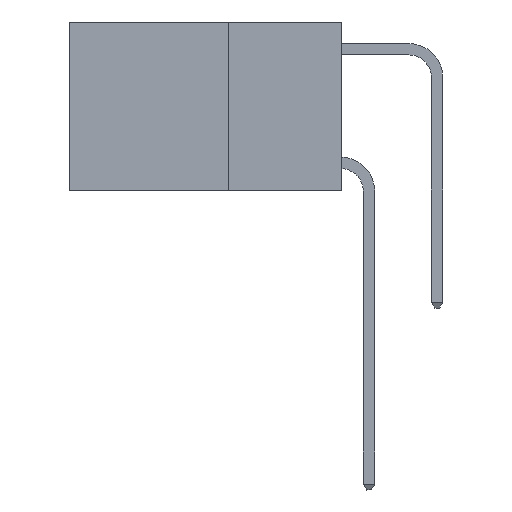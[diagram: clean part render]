
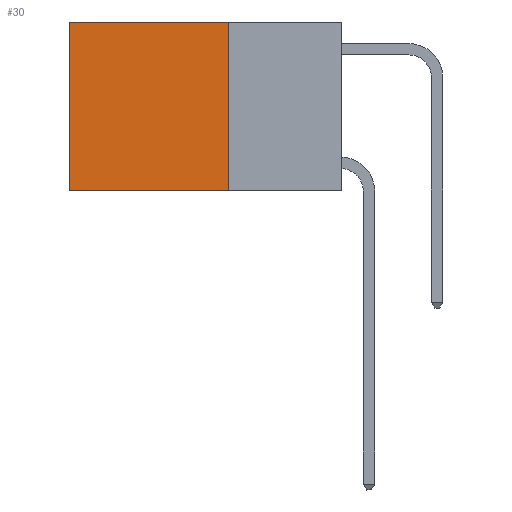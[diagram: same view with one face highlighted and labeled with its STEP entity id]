
A CAD part, left-side view. The second image highlights one B-rep face of the part: STEP entity #30.
In plain terms, the highlighted planar face has unit normal (-1, 0, 0).
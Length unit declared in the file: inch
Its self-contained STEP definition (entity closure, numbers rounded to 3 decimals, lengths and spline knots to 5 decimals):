
#30 = ADVANCED_FACE ( 'NONE', ( #6235 ), #3145, .F. ) ;
#73 = CARTESIAN_POINT ( 'NONE',  ( 0.2625, 0.25, 0. ) ) ;
#166 = DIRECTION ( 'NONE',  ( 1., 0., 0. ) ) ;
#639 = ORIENTED_EDGE ( 'NONE', *, *, #18662, .F. ) ;
#1713 = AXIS2_PLACEMENT_3D ( 'NONE', #73, #166, #11077 ) ;
#2638 = EDGE_CURVE ( 'NONE', #12230, #5429, #14148, .T. ) ;
#2720 = VERTEX_POINT ( 'NONE', #3259 ) ;
#3145 = PLANE ( 'NONE',  #1713 ) ;
#3259 = CARTESIAN_POINT ( 'NONE',  ( 0.2625, 0.6, -0.37 ) ) ;
#3732 = ORIENTED_EDGE ( 'NONE', *, *, #18533, .T. ) ;
#4660 = LINE ( 'NONE', #8150, #9643 ) ;
#4895 = ORIENTED_EDGE ( 'NONE', *, *, #7641, .F. ) ;
#5124 = LINE ( 'NONE', #6735, #8877 ) ;
#5429 = VERTEX_POINT ( 'NONE', #7804 ) ;
#6158 = DIRECTION ( 'NONE',  ( 0., 0., -1. ) ) ;
#6235 = FACE_OUTER_BOUND ( 'NONE', #14044, .T. ) ;
#6243 = CARTESIAN_POINT ( 'NONE',  ( 0.2625, 0.25, 0. ) ) ;
#6735 = CARTESIAN_POINT ( 'NONE',  ( 0.2625, 0.25, -0.37 ) ) ;
#7641 = EDGE_CURVE ( 'NONE', #12230, #20530, #4660, .T. ) ;
#7804 = CARTESIAN_POINT ( 'NONE',  ( 0.2625, 0.6, 0. ) ) ;
#8150 = CARTESIAN_POINT ( 'NONE',  ( 0.2625, 0.25, 0. ) ) ;
#8877 = VECTOR ( 'NONE', #16407, 39.37008 ) ;
#9643 = VECTOR ( 'NONE', #6158, 39.37008 ) ;
#10975 = DIRECTION ( 'NONE',  ( 0., 1., 0. ) ) ;
#11077 = DIRECTION ( 'NONE',  ( 0., 0., -1. ) ) ;
#12024 = ORIENTED_EDGE ( 'NONE', *, *, #2638, .T. ) ;
#12230 = VERTEX_POINT ( 'NONE', #13907 ) ;
#12534 = LINE ( 'NONE', #19246, #18949 ) ;
#13907 = CARTESIAN_POINT ( 'NONE',  ( 0.2625, 0.25, 0. ) ) ;
#14044 = EDGE_LOOP ( 'NONE', ( #3732, #639, #4895, #12024 ) ) ;
#14148 = LINE ( 'NONE', #6243, #15136 ) ;
#15136 = VECTOR ( 'NONE', #10975, 39.37008 ) ;
#16275 = CARTESIAN_POINT ( 'NONE',  ( 0.2625, 0.25, -0.37 ) ) ;
#16407 = DIRECTION ( 'NONE',  ( 0., 1., 0. ) ) ;
#17777 = DIRECTION ( 'NONE',  ( 0., 0., -1. ) ) ;
#18533 = EDGE_CURVE ( 'NONE', #5429, #2720, #12534, .T. ) ;
#18662 = EDGE_CURVE ( 'NONE', #20530, #2720, #5124, .T. ) ;
#18949 = VECTOR ( 'NONE', #17777, 39.37008 ) ;
#19246 = CARTESIAN_POINT ( 'NONE',  ( 0.2625, 0.6, 0. ) ) ;
#20530 = VERTEX_POINT ( 'NONE', #16275 ) ;
